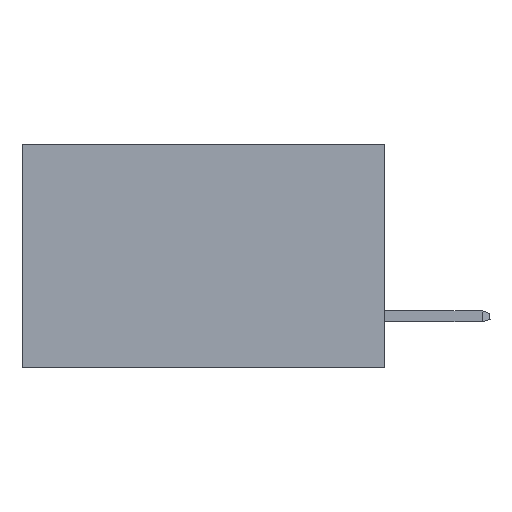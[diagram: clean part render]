
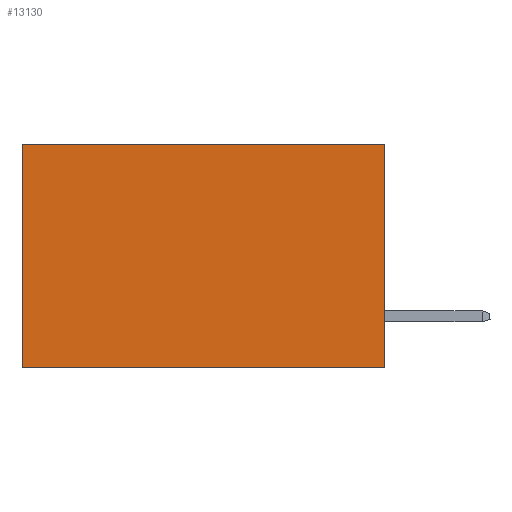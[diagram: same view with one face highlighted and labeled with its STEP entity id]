
A CAD part, left-side view. The second image highlights one B-rep face of the part: STEP entity #13130.
In plain terms, the highlighted planar face has unit normal (-1, 0, 0).
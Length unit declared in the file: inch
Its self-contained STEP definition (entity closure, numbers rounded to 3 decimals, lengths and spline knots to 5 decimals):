
#895 = AXIS2_PLACEMENT_3D ( 'NONE', #11166, #7795, #13643 ) ;
#1227 = VERTEX_POINT ( 'NONE', #8828 ) ;
#1631 = DIRECTION ( 'NONE',  ( 0., 1., 0. ) ) ;
#1667 = ORIENTED_EDGE ( 'NONE', *, *, #7132, .T. ) ;
#2033 = VECTOR ( 'NONE', #1631, 39.37008 ) ;
#2116 = DIRECTION ( 'NONE',  ( 0., 0., -1. ) ) ;
#2399 = VERTEX_POINT ( 'NONE', #13511 ) ;
#2695 = CARTESIAN_POINT ( 'NONE',  ( 0.298, 0., -0.37 ) ) ;
#2835 = ORIENTED_EDGE ( 'NONE', *, *, #13910, .F. ) ;
#3241 = VECTOR ( 'NONE', #3901, 39.37008 ) ;
#3372 = CARTESIAN_POINT ( 'NONE',  ( 0.298, 0., 0. ) ) ;
#3649 = DIRECTION ( 'NONE',  ( 0., 1., 0. ) ) ;
#3901 = DIRECTION ( 'NONE',  ( 0., 0., -1. ) ) ;
#5025 = CARTESIAN_POINT ( 'NONE',  ( 0.298, 0.6, -0.37 ) ) ;
#5067 = LINE ( 'NONE', #14094, #9400 ) ;
#5317 = LINE ( 'NONE', #2695, #2033 ) ;
#5727 = EDGE_LOOP ( 'NONE', ( #7458, #12097, #2835, #1667 ) ) ;
#6689 = LINE ( 'NONE', #7491, #3241 ) ;
#7132 = EDGE_CURVE ( 'NONE', #8935, #2399, #5067, .T. ) ;
#7171 = EDGE_CURVE ( 'NONE', #2399, #9688, #6689, .T. ) ;
#7458 = ORIENTED_EDGE ( 'NONE', *, *, #7171, .T. ) ;
#7491 = CARTESIAN_POINT ( 'NONE',  ( 0.298, 0.6, 0. ) ) ;
#7795 = DIRECTION ( 'NONE',  ( 1., 0., 0. ) ) ;
#8828 = CARTESIAN_POINT ( 'NONE',  ( 0.298, 0., -0.37 ) ) ;
#8935 = VERTEX_POINT ( 'NONE', #13867 ) ;
#9400 = VECTOR ( 'NONE', #3649, 39.37008 ) ;
#9606 = VECTOR ( 'NONE', #2116, 39.37008 ) ;
#9688 = VERTEX_POINT ( 'NONE', #5025 ) ;
#10905 = FACE_OUTER_BOUND ( 'NONE', #5727, .T. ) ;
#11166 = CARTESIAN_POINT ( 'NONE',  ( 0.298, 0., 0. ) ) ;
#12097 = ORIENTED_EDGE ( 'NONE', *, *, #13798, .F. ) ;
#12303 = PLANE ( 'NONE',  #895 ) ;
#12677 = LINE ( 'NONE', #3372, #9606 ) ;
#13130 = ADVANCED_FACE ( 'NONE', ( #10905 ), #12303, .F. ) ;
#13511 = CARTESIAN_POINT ( 'NONE',  ( 0.298, 0.6, 0. ) ) ;
#13643 = DIRECTION ( 'NONE',  ( 0., 0., -1. ) ) ;
#13798 = EDGE_CURVE ( 'NONE', #1227, #9688, #5317, .T. ) ;
#13867 = CARTESIAN_POINT ( 'NONE',  ( 0.298, 0., 0. ) ) ;
#13910 = EDGE_CURVE ( 'NONE', #8935, #1227, #12677, .T. ) ;
#14094 = CARTESIAN_POINT ( 'NONE',  ( 0.298, 0., 0. ) ) ;
